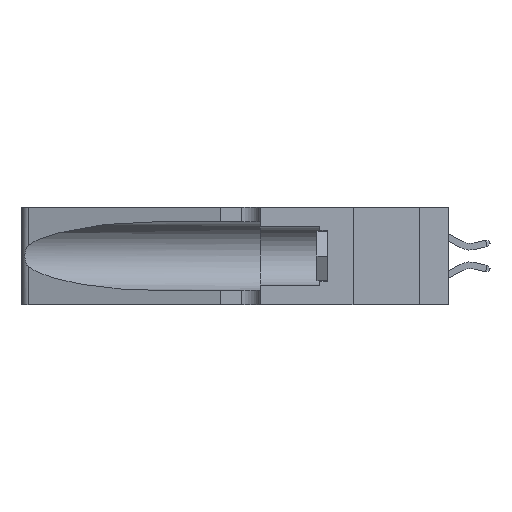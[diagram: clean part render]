
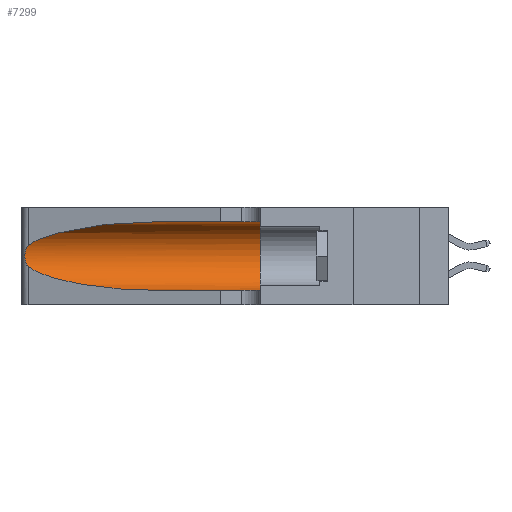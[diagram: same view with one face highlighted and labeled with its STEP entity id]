
A CAD part, left-side view. The second image highlights one B-rep face of the part: STEP entity #7299.
In plain terms, the highlighted cylindrical face has radius 3.308 mm (diameter 6.617 mm), a partial arc.
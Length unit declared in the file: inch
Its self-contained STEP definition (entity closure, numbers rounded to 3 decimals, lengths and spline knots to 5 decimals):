
#628 = CARTESIAN_POINT ( 'NONE',  ( 0.25487, 1.22718, 0.22369 ) ) ;
#725 = CARTESIAN_POINT ( 'NONE',  ( 0.25639, 1.23186, 0.15144 ) ) ;
#1280 = ORIENTED_EDGE ( 'NONE', *, *, #16436, .T. ) ;
#1346 = CARTESIAN_POINT ( 'NONE',  ( 0.1305, 0.72297, 0.05475 ) ) ;
#1698 = EDGE_CURVE ( 'NONE', #13113, #7789, #15404, .T. ) ;
#2215 = VERTEX_POINT ( 'NONE', #17298 ) ;
#3001 = CARTESIAN_POINT ( 'NONE',  ( 0.25487, 1.22718, 0.14631 ) ) ;
#3251 = VERTEX_POINT ( 'NONE', #16065 ) ;
#4950 = CARTESIAN_POINT ( 'NONE',  ( 0.1305, 0.72297, 0.31525 ) ) ;
#5006 = EDGE_CURVE ( 'NONE', #5970, #7789, #10811, .T. ) ;
#5188 = B_SPLINE_CURVE_WITH_KNOTS ( 'NONE', 3,
 ( #628, #18655, #5192, #20866, #7438, #23096, #9697, #25307, #11948, #27538, #14240, #725, #16517, #3001 ),
 .UNSPECIFIED., .F., .F.,
 ( 4, 2, 2, 2, 2, 2, 4 ),
 ( 0., 0.00027, 0.00053, 0.00107, 0.0016, 0.00187, 0.00214 ),
 .UNSPECIFIED. ) ;
#5192 = CARTESIAN_POINT ( 'NONE',  ( 0.25639, 1.23184, 0.21858 ) ) ;
#5970 = VERTEX_POINT ( 'NONE', #1346 ) ;
#6570 = ORIENTED_EDGE ( 'NONE', *, *, #5006, .T. ) ;
#6630 = ORIENTED_EDGE ( 'NONE', *, *, #27396, .T. ) ;
#7299 = ADVANCED_FACE ( 'NONE', ( #7557 ), #18815, .F. ) ;
#7438 = CARTESIAN_POINT ( 'NONE',  ( 0.25854, 1.2359, 0.20912 ) ) ;
#7440 = AXIS2_PLACEMENT_3D ( 'NONE', #17811, #20420, #28831 ) ;
#7557 = FACE_OUTER_BOUND ( 'NONE', #20148, .T. ) ;
#7789 = VERTEX_POINT ( 'NONE', #8829 ) ;
#8555 = CARTESIAN_POINT ( 'NONE',  ( 0.18966, 0.96281, 0.05475 ) ) ;
#8829 = CARTESIAN_POINT ( 'NONE',  ( 0.1305, 0.35, 0.05475 ) ) ;
#8840 = DIRECTION ( 'NONE',  ( 0., 1., 0. ) ) ;
#9697 = CARTESIAN_POINT ( 'NONE',  ( 0.26075, 1.23896, 0.19203 ) ) ;
#10811 = LINE ( 'NONE', #11042, #21314 ) ;
#11042 = CARTESIAN_POINT ( 'NONE',  ( 0.1305, 1.61858, 0.05475 ) ) ;
#11948 = CARTESIAN_POINT ( 'NONE',  ( 0.26017, 1.23833, 0.17102 ) ) ;
#12050 = CARTESIAN_POINT ( 'NONE',  ( 0.25487, 1.22718, 0.22369 ) ) ;
#12571 =( BOUNDED_CURVE ( )  B_SPLINE_CURVE ( 3, ( #4950, #18401, #27277, #13979 ),
 .UNSPECIFIED., .F., .T. ) 
 B_SPLINE_CURVE_WITH_KNOTS ( ( 4, 4 ),
 ( 1.5708, 2.84003 ),
 .UNSPECIFIED. ) 
 CURVE ( )  GEOMETRIC_REPRESENTATION_ITEM ( )  RATIONAL_B_SPLINE_CURVE ( ( 1., 0.87, 0.87, 1. ) ) 
 REPRESENTATION_ITEM ( '' )  );
#13113 = VERTEX_POINT ( 'NONE', #27175 ) ;
#13945 = LINE ( 'NONE', #19750, #25079 ) ;
#13979 = CARTESIAN_POINT ( 'NONE',  ( 0.25487, 1.22718, 0.22369 ) ) ;
#14240 = CARTESIAN_POINT ( 'NONE',  ( 0.25789, 1.23486, 0.15765 ) ) ;
#15273 = ORIENTED_EDGE ( 'NONE', *, *, #1698, .F. ) ;
#15404 = CIRCLE ( 'NONE', #19430, 0.13025 ) ;
#16009 = ORIENTED_EDGE ( 'NONE', *, *, #27070, .T. ) ;
#16065 = CARTESIAN_POINT ( 'NONE',  ( 0.25487, 1.22718, 0.14631 ) ) ;
#16436 = EDGE_CURVE ( 'NONE', #2215, #28985, #12571, .T. ) ;
#16517 = CARTESIAN_POINT ( 'NONE',  ( 0.25555, 1.22993, 0.14849 ) ) ;
#17298 = CARTESIAN_POINT ( 'NONE',  ( 0.1305, 0.72297, 0.31525 ) ) ;
#17811 = CARTESIAN_POINT ( 'NONE',  ( 0.1305, 1.61858, 0.185 ) ) ;
#18401 = CARTESIAN_POINT ( 'NONE',  ( 0.18966, 0.96281, 0.31525 ) ) ;
#18655 = CARTESIAN_POINT ( 'NONE',  ( 0.25555, 1.22994, 0.2215 ) ) ;
#18815 = CYLINDRICAL_SURFACE ( 'NONE', #7440, 0.13025 ) ;
#19430 = AXIS2_PLACEMENT_3D ( 'NONE', #22256, #8840, #24481 ) ;
#19750 = CARTESIAN_POINT ( 'NONE',  ( 0.1305, 1.61858, 0.31525 ) ) ;
#19751 = CARTESIAN_POINT ( 'NONE',  ( 0.25487, 1.22718, 0.14631 ) ) ;
#20148 = EDGE_LOOP ( 'NONE', ( #1280, #6630, #16009, #6570, #15273, #20679 ) ) ;
#20420 = DIRECTION ( 'NONE',  ( 0., -1., 0. ) ) ;
#20679 = ORIENTED_EDGE ( 'NONE', *, *, #28608, .F. ) ;
#20815 =( BOUNDED_CURVE ( )  B_SPLINE_CURVE ( 3, ( #19751, #21961, #8555, #24203 ),
 .UNSPECIFIED., .F., .F. ) 
 B_SPLINE_CURVE_WITH_KNOTS ( ( 4, 4 ),
 ( 3.44316, 4.71239 ),
 .UNSPECIFIED. ) 
 CURVE ( )  GEOMETRIC_REPRESENTATION_ITEM ( )  RATIONAL_B_SPLINE_CURVE ( ( 1., 0.87, 0.87, 1. ) ) 
 REPRESENTATION_ITEM ( '' )  );
#20866 = CARTESIAN_POINT ( 'NONE',  ( 0.25787, 1.23484, 0.2124 ) ) ;
#21314 = VECTOR ( 'NONE', #24437, 39.37008 ) ;
#21961 = CARTESIAN_POINT ( 'NONE',  ( 0.2373, 1.15595, 0.08982 ) ) ;
#22256 = CARTESIAN_POINT ( 'NONE',  ( 0.1305, 0.35, 0.185 ) ) ;
#23096 = CARTESIAN_POINT ( 'NONE',  ( 0.26018, 1.23835, 0.19895 ) ) ;
#24203 = CARTESIAN_POINT ( 'NONE',  ( 0.1305, 0.72297, 0.05475 ) ) ;
#24437 = DIRECTION ( 'NONE',  ( 0., -1., 0. ) ) ;
#24481 = DIRECTION ( 'NONE',  ( 0., 0., 1. ) ) ;
#25079 = VECTOR ( 'NONE', #28641, 39.37008 ) ;
#25307 = CARTESIAN_POINT ( 'NONE',  ( 0.26075, 1.23896, 0.178 ) ) ;
#27070 = EDGE_CURVE ( 'NONE', #3251, #5970, #20815, .T. ) ;
#27175 = CARTESIAN_POINT ( 'NONE',  ( 0.1305, 0.35, 0.31525 ) ) ;
#27277 = CARTESIAN_POINT ( 'NONE',  ( 0.2373, 1.15595, 0.28018 ) ) ;
#27396 = EDGE_CURVE ( 'NONE', #28985, #3251, #5188, .T. ) ;
#27538 = CARTESIAN_POINT ( 'NONE',  ( 0.25856, 1.23593, 0.16098 ) ) ;
#28608 = EDGE_CURVE ( 'NONE', #2215, #13113, #13945, .T. ) ;
#28641 = DIRECTION ( 'NONE',  ( 0., -1., 0. ) ) ;
#28831 = DIRECTION ( 'NONE',  ( 0., 0., -1. ) ) ;
#28985 = VERTEX_POINT ( 'NONE', #12050 ) ;
